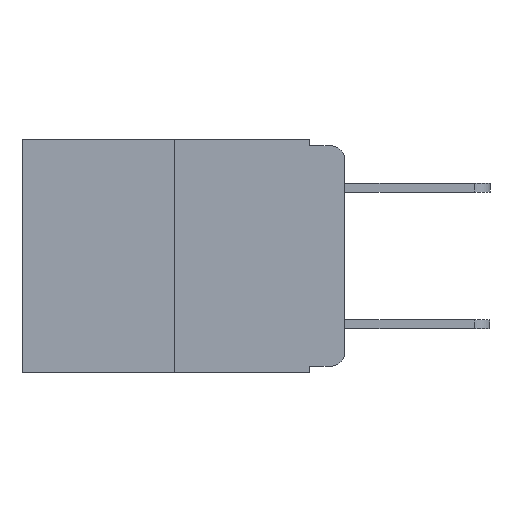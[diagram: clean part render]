
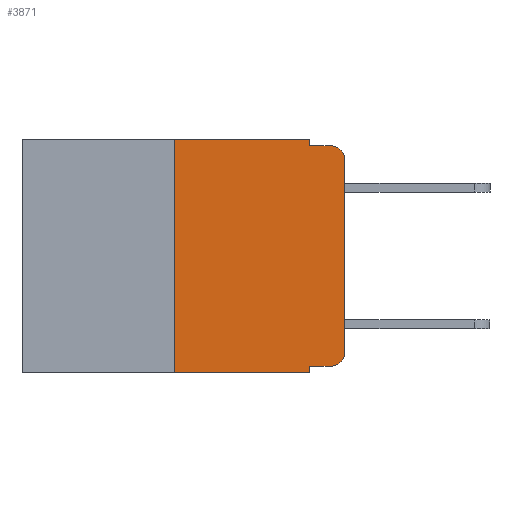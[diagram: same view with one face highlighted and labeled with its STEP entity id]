
A CAD part, left-side view. The second image highlights one B-rep face of the part: STEP entity #3871.
In plain terms, the highlighted planar face has unit normal (-1, 0, 0).
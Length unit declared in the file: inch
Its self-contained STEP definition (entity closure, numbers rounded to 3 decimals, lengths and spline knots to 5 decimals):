
#152 = ORIENTED_EDGE ( 'NONE', *, *, #24915, .F. ) ;
#622 = CIRCLE ( 'NONE', #19036, 0.02 ) ;
#1043 = VERTEX_POINT ( 'NONE', #1129 ) ;
#1129 = CARTESIAN_POINT ( 'NONE',  ( 0., 0., -0.03 ) ) ;
#1298 = VERTEX_POINT ( 'NONE', #21232 ) ;
#1509 = VECTOR ( 'NONE', #3308, 39.37008 ) ;
#2611 = VERTEX_POINT ( 'NONE', #4461 ) ;
#3112 = VECTOR ( 'NONE', #3688, 39.37008 ) ;
#3308 = DIRECTION ( 'NONE',  ( 0., -1., 0. ) ) ;
#3386 = VERTEX_POINT ( 'NONE', #8856 ) ;
#3671 = CARTESIAN_POINT ( 'NONE',  ( 0., 0.473, -0.343 ) ) ;
#3688 = DIRECTION ( 'NONE',  ( 0., -1., 0. ) ) ;
#3745 = ORIENTED_EDGE ( 'NONE', *, *, #10929, .F. ) ;
#3871 = ADVANCED_FACE ( 'NONE', ( #13894 ), #12465, .F. ) ;
#4208 = DIRECTION ( 'NONE',  ( 0., 0., -1. ) ) ;
#4461 = CARTESIAN_POINT ( 'NONE',  ( 0., 0., -0.313 ) ) ;
#4669 = LINE ( 'NONE', #16537, #13811 ) ;
#4675 = DIRECTION ( 'NONE',  ( -1., 0., 0. ) ) ;
#4973 = VERTEX_POINT ( 'NONE', #26384 ) ;
#5062 = CARTESIAN_POINT ( 'NONE',  ( 0., 0.051, -0.343 ) ) ;
#5842 = CARTESIAN_POINT ( 'NONE',  ( 0., 0.051, -0.01 ) ) ;
#5932 = AXIS2_PLACEMENT_3D ( 'NONE', #8407, #16668, #4208 ) ;
#5945 = CARTESIAN_POINT ( 'NONE',  ( 0., 0.051, 0. ) ) ;
#6233 = EDGE_CURVE ( 'NONE', #8093, #20267, #23429, .T. ) ;
#6595 = VERTEX_POINT ( 'NONE', #15354 ) ;
#6758 = EDGE_CURVE ( 'NONE', #6595, #4973, #16233, .T. ) ;
#6853 = ORIENTED_EDGE ( 'NONE', *, *, #9415, .F. ) ;
#6973 = VECTOR ( 'NONE', #8070, 39.37008 ) ;
#7091 = ORIENTED_EDGE ( 'NONE', *, *, #6233, .F. ) ;
#7582 = LINE ( 'NONE', #5945, #17866 ) ;
#7880 = ORIENTED_EDGE ( 'NONE', *, *, #6758, .F. ) ;
#8052 = AXIS2_PLACEMENT_3D ( 'NONE', #8864, #23034, #10943 ) ;
#8070 = DIRECTION ( 'NONE',  ( 0., -1., 0. ) ) ;
#8093 = VERTEX_POINT ( 'NONE', #5842 ) ;
#8095 = DIRECTION ( 'NONE',  ( 0., 0., -1. ) ) ;
#8407 = CARTESIAN_POINT ( 'NONE',  ( 0., 0.473, 0. ) ) ;
#8856 = CARTESIAN_POINT ( 'NONE',  ( 0., 0.051, 0. ) ) ;
#8864 = CARTESIAN_POINT ( 'NONE',  ( 0., 0.02, -0.313 ) ) ;
#9415 = EDGE_CURVE ( 'NONE', #4973, #3386, #18992, .T. ) ;
#10751 = VECTOR ( 'NONE', #15885, 39.37008 ) ;
#10782 = ORIENTED_EDGE ( 'NONE', *, *, #11871, .T. ) ;
#10929 = EDGE_CURVE ( 'NONE', #3386, #8093, #22004, .T. ) ;
#10943 = DIRECTION ( 'NONE',  ( 0., 0., -1. ) ) ;
#11740 = VERTEX_POINT ( 'NONE', #19846 ) ;
#11871 = EDGE_CURVE ( 'NONE', #6595, #18673, #18533, .T. ) ;
#12465 = PLANE ( 'NONE',  #5932 ) ;
#12506 = DIRECTION ( 'NONE',  ( 0., -1., 0. ) ) ;
#13313 = EDGE_CURVE ( 'NONE', #11740, #2611, #15656, .T. ) ;
#13811 = VECTOR ( 'NONE', #12506, 39.37008 ) ;
#13820 = CARTESIAN_POINT ( 'NONE',  ( 0., 0.25, 0. ) ) ;
#13894 = FACE_OUTER_BOUND ( 'NONE', #23275, .T. ) ;
#15354 = CARTESIAN_POINT ( 'NONE',  ( 0., 0.25, -0.343 ) ) ;
#15656 = CIRCLE ( 'NONE', #8052, 0.02 ) ;
#15885 = DIRECTION ( 'NONE',  ( 0., 0., 1. ) ) ;
#15936 = EDGE_CURVE ( 'NONE', #1043, #20267, #622, .T. ) ;
#16070 = VECTOR ( 'NONE', #23855, 39.37008 ) ;
#16187 = CARTESIAN_POINT ( 'NONE',  ( 0., 0.473, 0. ) ) ;
#16233 = LINE ( 'NONE', #13820, #10751 ) ;
#16537 = CARTESIAN_POINT ( 'NONE',  ( 0., 0.051, -0.333 ) ) ;
#16668 = DIRECTION ( 'NONE',  ( 1., 0., 0. ) ) ;
#17037 = CARTESIAN_POINT ( 'NONE',  ( 0., 0., 0. ) ) ;
#17131 = CARTESIAN_POINT ( 'NONE',  ( 0., 0.02, -0.03 ) ) ;
#17866 = VECTOR ( 'NONE', #8095, 39.37008 ) ;
#18236 = VECTOR ( 'NONE', #24906, 39.37008 ) ;
#18533 = LINE ( 'NONE', #3671, #6973 ) ;
#18673 = VERTEX_POINT ( 'NONE', #5062 ) ;
#18992 = LINE ( 'NONE', #16187, #3112 ) ;
#19036 = AXIS2_PLACEMENT_3D ( 'NONE', #17131, #4675, #19109 ) ;
#19109 = DIRECTION ( 'NONE',  ( 0., 0., -1. ) ) ;
#19846 = CARTESIAN_POINT ( 'NONE',  ( 0., 0.02, -0.333 ) ) ;
#19854 = CARTESIAN_POINT ( 'NONE',  ( 0., 0.051, -0.01 ) ) ;
#20267 = VERTEX_POINT ( 'NONE', #25225 ) ;
#20996 = ORIENTED_EDGE ( 'NONE', *, *, #23229, .T. ) ;
#21232 = CARTESIAN_POINT ( 'NONE',  ( 0., 0.051, -0.333 ) ) ;
#21877 = CARTESIAN_POINT ( 'NONE',  ( 0., 0.051, 0. ) ) ;
#22004 = LINE ( 'NONE', #21877, #16070 ) ;
#23034 = DIRECTION ( 'NONE',  ( -1., 0., 0. ) ) ;
#23229 = EDGE_CURVE ( 'NONE', #1298, #11740, #4669, .T. ) ;
#23275 = EDGE_LOOP ( 'NONE', ( #23574, #24799, #7091, #3745, #6853, #7880, #10782, #152, #20996, #24720 ) ) ;
#23429 = LINE ( 'NONE', #19854, #1509 ) ;
#23493 = LINE ( 'NONE', #17037, #18236 ) ;
#23574 = ORIENTED_EDGE ( 'NONE', *, *, #23945, .T. ) ;
#23855 = DIRECTION ( 'NONE',  ( 0., 0., -1. ) ) ;
#23945 = EDGE_CURVE ( 'NONE', #2611, #1043, #23493, .T. ) ;
#24720 = ORIENTED_EDGE ( 'NONE', *, *, #13313, .T. ) ;
#24799 = ORIENTED_EDGE ( 'NONE', *, *, #15936, .T. ) ;
#24906 = DIRECTION ( 'NONE',  ( 0., 0., 1. ) ) ;
#24915 = EDGE_CURVE ( 'NONE', #1298, #18673, #7582, .T. ) ;
#25225 = CARTESIAN_POINT ( 'NONE',  ( 0., 0.02, -0.01 ) ) ;
#26384 = CARTESIAN_POINT ( 'NONE',  ( 0., 0.25, 0. ) ) ;
